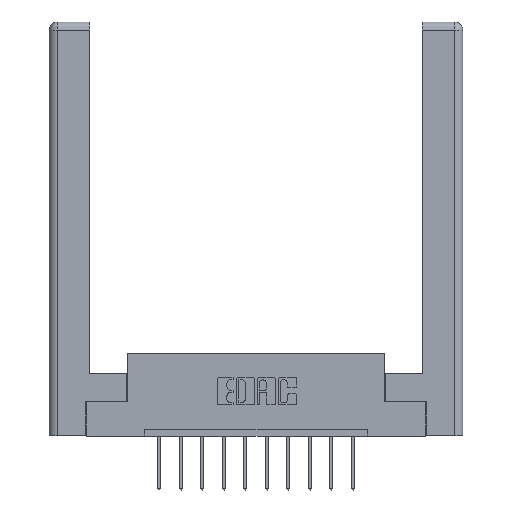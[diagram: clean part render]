
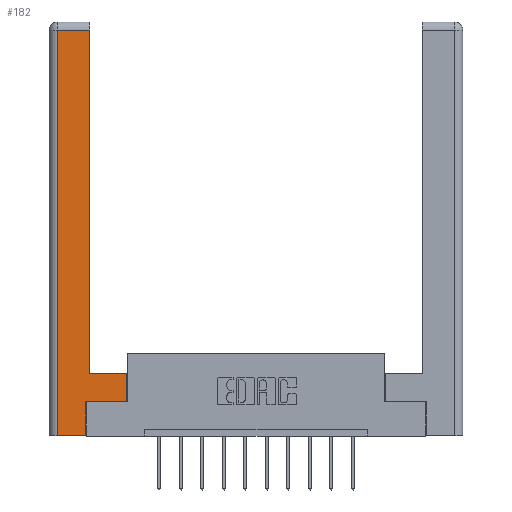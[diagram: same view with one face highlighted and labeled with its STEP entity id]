
A CAD part, top view. The second image highlights one B-rep face of the part: STEP entity #182.
In plain terms, the highlighted planar face has unit normal (0, 0, 1).
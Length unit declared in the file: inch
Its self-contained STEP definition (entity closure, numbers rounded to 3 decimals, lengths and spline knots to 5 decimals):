
#57 = VECTOR ( 'NONE', #2452, 39.37008 ) ;
#71 = VECTOR ( 'NONE', #10626, 39.37008 ) ;
#182 = ADVANCED_FACE ( 'NONE', ( #4778 ), #406, .F. ) ;
#243 = CARTESIAN_POINT ( 'NONE',  ( 0.295, 3., 0. ) ) ;
#258 = DIRECTION ( 'NONE',  ( 0., 0., -1. ) ) ;
#299 = DIRECTION ( 'NONE',  ( 0., 1., 0. ) ) ;
#406 = PLANE ( 'NONE',  #4129 ) ;
#630 = VECTOR ( 'NONE', #13169, 39.37008 ) ;
#1120 = EDGE_CURVE ( 'NONE', #8807, #2149, #11804, .T. ) ;
#1549 = VERTEX_POINT ( 'NONE', #6270 ) ;
#2093 = ORIENTED_EDGE ( 'NONE', *, *, #8355, .T. ) ;
#2149 = VERTEX_POINT ( 'NONE', #3049 ) ;
#2452 = DIRECTION ( 'NONE',  ( 0., -1., 0. ) ) ;
#2644 = ORIENTED_EDGE ( 'NONE', *, *, #6901, .T. ) ;
#2678 = LINE ( 'NONE', #12095, #630 ) ;
#2949 = VERTEX_POINT ( 'NONE', #6986 ) ;
#2958 = VERTEX_POINT ( 'NONE', #9251 ) ;
#3032 = CARTESIAN_POINT ( 'NONE',  ( 0.295, 0.45, 0. ) ) ;
#3049 = CARTESIAN_POINT ( 'NONE',  ( 0.265, 0., 0. ) ) ;
#3778 = CARTESIAN_POINT ( 'NONE',  ( 0.0615, 0., 0. ) ) ;
#3904 = EDGE_CURVE ( 'NONE', #11946, #2958, #8174, .T. ) ;
#4080 = ORIENTED_EDGE ( 'NONE', *, *, #8986, .T. ) ;
#4129 = AXIS2_PLACEMENT_3D ( 'NONE', #13421, #258, #12305 ) ;
#4687 = EDGE_CURVE ( 'NONE', #1549, #6543, #2678, .T. ) ;
#4778 = FACE_OUTER_BOUND ( 'NONE', #7176, .T. ) ;
#5334 = ORIENTED_EDGE ( 'NONE', *, *, #13940, .T. ) ;
#6270 = CARTESIAN_POINT ( 'NONE',  ( 0.565, 0.45, 0. ) ) ;
#6483 = VERTEX_POINT ( 'NONE', #14010 ) ;
#6489 = ORIENTED_EDGE ( 'NONE', *, *, #1120, .T. ) ;
#6543 = VERTEX_POINT ( 'NONE', #3032 ) ;
#6546 = DIRECTION ( 'NONE',  ( 0., 1., 0. ) ) ;
#6561 = LINE ( 'NONE', #243, #8260 ) ;
#6584 = DIRECTION ( 'NONE',  ( 1., 0., 0. ) ) ;
#6768 = LINE ( 'NONE', #9012, #57 ) ;
#6901 = EDGE_CURVE ( 'NONE', #2958, #8807, #6768, .T. ) ;
#6986 = CARTESIAN_POINT ( 'NONE',  ( 0.265, 0.245, 0. ) ) ;
#7176 = EDGE_LOOP ( 'NONE', ( #2093, #10800, #2644, #6489, #5334, #4080, #13683, #13261 ) ) ;
#8174 = LINE ( 'NONE', #13863, #71 ) ;
#8260 = VECTOR ( 'NONE', #299, 39.37008 ) ;
#8355 = EDGE_CURVE ( 'NONE', #6543, #11946, #6561, .T. ) ;
#8531 = LINE ( 'NONE', #9819, #13318 ) ;
#8807 = VERTEX_POINT ( 'NONE', #3778 ) ;
#8986 = EDGE_CURVE ( 'NONE', #2949, #6483, #11195, .T. ) ;
#9012 = CARTESIAN_POINT ( 'NONE',  ( 0.0615, 0., 0. ) ) ;
#9079 = CARTESIAN_POINT ( 'NONE',  ( 0.295, 2.94, 0. ) ) ;
#9251 = CARTESIAN_POINT ( 'NONE',  ( 0.0615, 2.94, 0. ) ) ;
#9668 = VECTOR ( 'NONE', #6584, 39.37008 ) ;
#9819 = CARTESIAN_POINT ( 'NONE',  ( 0.565, 0.45, 0. ) ) ;
#10067 = CARTESIAN_POINT ( 'NONE',  ( 0.265, 0.245, 0. ) ) ;
#10484 = EDGE_CURVE ( 'NONE', #6483, #1549, #8531, .T. ) ;
#10626 = DIRECTION ( 'NONE',  ( -1., 0., 0. ) ) ;
#10800 = ORIENTED_EDGE ( 'NONE', *, *, #3904, .T. ) ;
#11035 = VECTOR ( 'NONE', #12087, 39.37008 ) ;
#11195 = LINE ( 'NONE', #13103, #9668 ) ;
#11804 = LINE ( 'NONE', #14238, #13843 ) ;
#11946 = VERTEX_POINT ( 'NONE', #9079 ) ;
#12071 = DIRECTION ( 'NONE',  ( 1., 0., 0. ) ) ;
#12087 = DIRECTION ( 'NONE',  ( 0., 1., 0. ) ) ;
#12095 = CARTESIAN_POINT ( 'NONE',  ( 0.295, 0.45, 0. ) ) ;
#12305 = DIRECTION ( 'NONE',  ( -1., 0., 0. ) ) ;
#12558 = LINE ( 'NONE', #10067, #11035 ) ;
#13103 = CARTESIAN_POINT ( 'NONE',  ( 0.565, 0.245, 0. ) ) ;
#13169 = DIRECTION ( 'NONE',  ( -1., 0., 0. ) ) ;
#13261 = ORIENTED_EDGE ( 'NONE', *, *, #4687, .T. ) ;
#13318 = VECTOR ( 'NONE', #6546, 39.37008 ) ;
#13421 = CARTESIAN_POINT ( 'NONE',  ( 0., 0., 0. ) ) ;
#13683 = ORIENTED_EDGE ( 'NONE', *, *, #10484, .T. ) ;
#13843 = VECTOR ( 'NONE', #12071, 39.37008 ) ;
#13863 = CARTESIAN_POINT ( 'NONE',  ( 0.0615, 2.94, 0. ) ) ;
#13940 = EDGE_CURVE ( 'NONE', #2149, #2949, #12558, .T. ) ;
#14010 = CARTESIAN_POINT ( 'NONE',  ( 0.565, 0.245, 0. ) ) ;
#14238 = CARTESIAN_POINT ( 'NONE',  ( 0.265, 0., 0. ) ) ;
